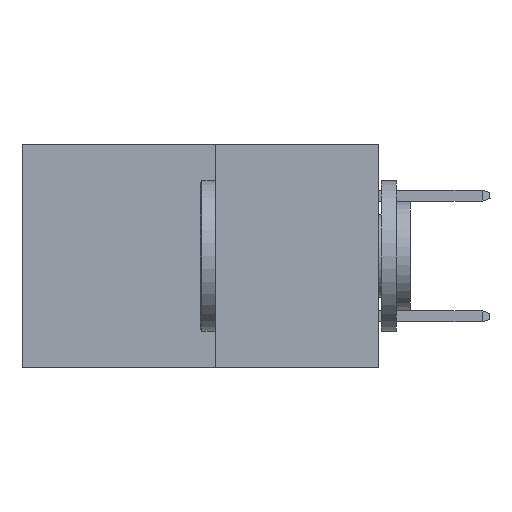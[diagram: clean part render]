
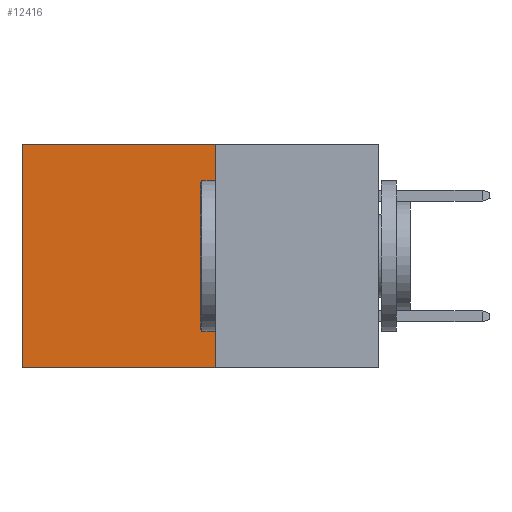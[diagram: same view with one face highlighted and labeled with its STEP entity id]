
A CAD part, left-side view. The second image highlights one B-rep face of the part: STEP entity #12416.
In plain terms, the highlighted planar face has unit normal (-1, 0, 0).
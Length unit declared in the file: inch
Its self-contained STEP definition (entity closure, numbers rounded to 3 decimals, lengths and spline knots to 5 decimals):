
#117 = VERTEX_POINT ( 'NONE', #10665 ) ;
#780 = LINE ( 'NONE', #18945, #26146 ) ;
#2298 = DIRECTION ( 'NONE',  ( 0., 0., -1. ) ) ;
#4996 = CARTESIAN_POINT ( 'NONE',  ( 0.277, 0.59, -0.37 ) ) ;
#5542 = VECTOR ( 'NONE', #11953, 39.37008 ) ;
#6940 = EDGE_LOOP ( 'NONE', ( #21958, #19541, #10643, #16815 ) ) ;
#8522 = EDGE_CURVE ( 'NONE', #29822, #12770, #780, .T. ) ;
#9473 = CARTESIAN_POINT ( 'NONE',  ( 0.277, 0.27, -0.37 ) ) ;
#10373 = VECTOR ( 'NONE', #19718, 39.37008 ) ;
#10638 = AXIS2_PLACEMENT_3D ( 'NONE', #31719, #17030, #2298 ) ;
#10643 = ORIENTED_EDGE ( 'NONE', *, *, #8522, .F. ) ;
#10665 = CARTESIAN_POINT ( 'NONE',  ( 0.277, 0.59, -0.37 ) ) ;
#10956 = CARTESIAN_POINT ( 'NONE',  ( 0.277, 0.27, -0.37 ) ) ;
#11668 = DIRECTION ( 'NONE',  ( 0., 0., -1. ) ) ;
#11727 = EDGE_CURVE ( 'NONE', #12770, #117, #25143, .T. ) ;
#11953 = DIRECTION ( 'NONE',  ( 0., 1., 0. ) ) ;
#12416 = ADVANCED_FACE ( 'NONE', ( #25843 ), #26694, .F. ) ;
#12711 = DIRECTION ( 'NONE',  ( 0., 1., 0. ) ) ;
#12770 = VERTEX_POINT ( 'NONE', #10956 ) ;
#13140 = LINE ( 'NONE', #29737, #13908 ) ;
#13908 = VECTOR ( 'NONE', #12711, 39.37008 ) ;
#14320 = EDGE_CURVE ( 'NONE', #22863, #117, #16873, .T. ) ;
#16815 = ORIENTED_EDGE ( 'NONE', *, *, #31190, .T. ) ;
#16873 = LINE ( 'NONE', #4996, #10373 ) ;
#17030 = DIRECTION ( 'NONE',  ( 1., 0., 0. ) ) ;
#18945 = CARTESIAN_POINT ( 'NONE',  ( 0.277, 0.27, -0.37 ) ) ;
#19085 = CARTESIAN_POINT ( 'NONE',  ( 0.277, 0.59, 0. ) ) ;
#19541 = ORIENTED_EDGE ( 'NONE', *, *, #11727, .F. ) ;
#19718 = DIRECTION ( 'NONE',  ( 0., 0., -1. ) ) ;
#21958 = ORIENTED_EDGE ( 'NONE', *, *, #14320, .T. ) ;
#22187 = CARTESIAN_POINT ( 'NONE',  ( 0.277, 0.27, 0. ) ) ;
#22863 = VERTEX_POINT ( 'NONE', #19085 ) ;
#25143 = LINE ( 'NONE', #9473, #5542 ) ;
#25843 = FACE_OUTER_BOUND ( 'NONE', #6940, .T. ) ;
#26146 = VECTOR ( 'NONE', #11668, 39.37008 ) ;
#26694 = PLANE ( 'NONE',  #10638 ) ;
#29737 = CARTESIAN_POINT ( 'NONE',  ( 0.277, 0.27, 0. ) ) ;
#29822 = VERTEX_POINT ( 'NONE', #22187 ) ;
#31190 = EDGE_CURVE ( 'NONE', #29822, #22863, #13140, .T. ) ;
#31719 = CARTESIAN_POINT ( 'NONE',  ( 0.277, 0.27, -0.37 ) ) ;
